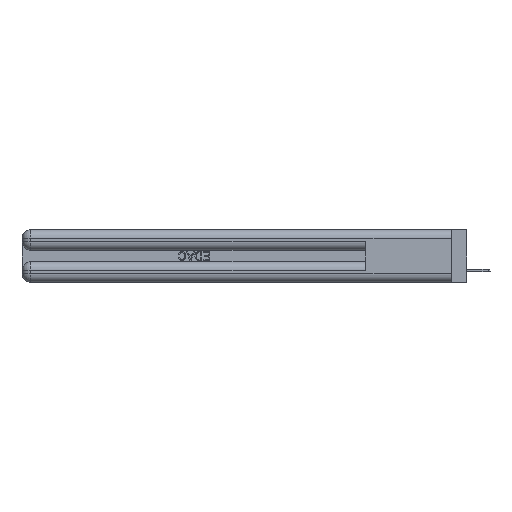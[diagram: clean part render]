
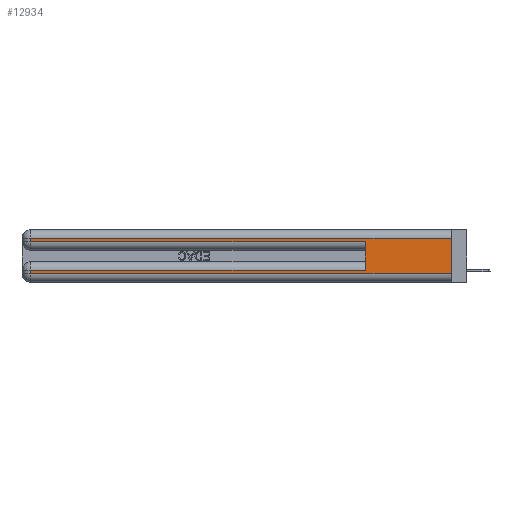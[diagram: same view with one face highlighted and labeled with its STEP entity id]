
A CAD part, left-side view. The second image highlights one B-rep face of the part: STEP entity #12934.
In plain terms, the highlighted planar face has unit normal (-1, 0, 0).
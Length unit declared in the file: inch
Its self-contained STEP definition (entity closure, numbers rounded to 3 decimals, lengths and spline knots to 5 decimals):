
#22 = AXIS2_PLACEMENT_3D ( 'NONE', #28005, #27720, #12625 ) ;
#767 = VECTOR ( 'NONE', #29640, 39.37008 ) ;
#1498 = CARTESIAN_POINT ( 'NONE',  ( 0., 0.6, 0.285 ) ) ;
#1683 = ORIENTED_EDGE ( 'NONE', *, *, #37408, .T. ) ;
#1996 = LINE ( 'NONE', #8530, #46665 ) ;
#2522 = CARTESIAN_POINT ( 'NONE',  ( 0., 0., 0.31 ) ) ;
#2991 = ORIENTED_EDGE ( 'NONE', *, *, #3383, .F. ) ;
#3135 = ORIENTED_EDGE ( 'NONE', *, *, #40833, .F. ) ;
#3327 = VECTOR ( 'NONE', #6158, 39.37008 ) ;
#3383 = EDGE_CURVE ( 'NONE', #21858, #6400, #47282, .T. ) ;
#4470 = LINE ( 'NONE', #31161, #49171 ) ;
#5567 = VERTEX_POINT ( 'NONE', #1498 ) ;
#6158 = DIRECTION ( 'NONE',  ( 0., 0., -1. ) ) ;
#6400 = VERTEX_POINT ( 'NONE', #17814 ) ;
#6963 = CARTESIAN_POINT ( 'NONE',  ( 0., 0.6, 0.145 ) ) ;
#8530 = CARTESIAN_POINT ( 'NONE',  ( 0., 2.94, 0.37 ) ) ;
#11016 = CARTESIAN_POINT ( 'NONE',  ( 0., 2.94, 0.37 ) ) ;
#11525 = CARTESIAN_POINT ( 'NONE',  ( 0., 2.94, 0.085 ) ) ;
#11971 = EDGE_CURVE ( 'NONE', #12400, #48151, #46925, .T. ) ;
#12214 = DIRECTION ( 'NONE',  ( 0., 0., -1. ) ) ;
#12400 = VERTEX_POINT ( 'NONE', #11525 ) ;
#12556 = ORIENTED_EDGE ( 'NONE', *, *, #29020, .T. ) ;
#12625 = DIRECTION ( 'NONE',  ( 0., 0., -1. ) ) ;
#12934 = ADVANCED_FACE ( 'NONE', ( #42698 ), #24465, .F. ) ;
#14293 = LINE ( 'NONE', #35962, #14870 ) ;
#14870 = VECTOR ( 'NONE', #16725, 39.37008 ) ;
#16725 = DIRECTION ( 'NONE',  ( 0., -1., 0. ) ) ;
#16782 = VECTOR ( 'NONE', #26331, 39.37008 ) ;
#17787 = LINE ( 'NONE', #41092, #767 ) ;
#17814 = CARTESIAN_POINT ( 'NONE',  ( 0., 0., 0.06 ) ) ;
#18888 = DIRECTION ( 'NONE',  ( 0., 0., -1. ) ) ;
#19220 = VECTOR ( 'NONE', #18888, 39.37008 ) ;
#21858 = VERTEX_POINT ( 'NONE', #2522 ) ;
#24045 = EDGE_CURVE ( 'NONE', #32483, #24258, #1996, .T. ) ;
#24258 = VERTEX_POINT ( 'NONE', #35124 ) ;
#24414 = DIRECTION ( 'NONE',  ( 0., 1., 0. ) ) ;
#24460 = LINE ( 'NONE', #47608, #30542 ) ;
#24465 = PLANE ( 'NONE',  #22 ) ;
#25417 = CARTESIAN_POINT ( 'NONE',  ( 0., 0., 0.37 ) ) ;
#25487 = EDGE_LOOP ( 'NONE', ( #2991, #12556, #35026, #29604, #3135, #1683, #39627, #26006 ) ) ;
#26006 = ORIENTED_EDGE ( 'NONE', *, *, #37090, .T. ) ;
#26331 = DIRECTION ( 'NONE',  ( 0., 0., 1. ) ) ;
#27024 = CARTESIAN_POINT ( 'NONE',  ( 0., 2.94, 0.06 ) ) ;
#27114 = LINE ( 'NONE', #6963, #16782 ) ;
#27720 = DIRECTION ( 'NONE',  ( 1., 0., 0. ) ) ;
#28005 = CARTESIAN_POINT ( 'NONE',  ( 0., 0., 0.37 ) ) ;
#29020 = EDGE_CURVE ( 'NONE', #21858, #32483, #4470, .T. ) ;
#29604 = ORIENTED_EDGE ( 'NONE', *, *, #37640, .T. ) ;
#29640 = DIRECTION ( 'NONE',  ( 0., -1., 0. ) ) ;
#30542 = VECTOR ( 'NONE', #24414, 39.37008 ) ;
#31161 = CARTESIAN_POINT ( 'NONE',  ( 0., 0., 0.31 ) ) ;
#32483 = VERTEX_POINT ( 'NONE', #37504 ) ;
#35026 = ORIENTED_EDGE ( 'NONE', *, *, #24045, .T. ) ;
#35077 = CARTESIAN_POINT ( 'NONE',  ( 0., 0.6, 0.085 ) ) ;
#35124 = CARTESIAN_POINT ( 'NONE',  ( 0., 2.94, 0.285 ) ) ;
#35163 = DIRECTION ( 'NONE',  ( 0., 1., 0. ) ) ;
#35962 = CARTESIAN_POINT ( 'NONE',  ( 0., 0., 0.06 ) ) ;
#37090 = EDGE_CURVE ( 'NONE', #48151, #6400, #14293, .T. ) ;
#37408 = EDGE_CURVE ( 'NONE', #42700, #12400, #24460, .T. ) ;
#37504 = CARTESIAN_POINT ( 'NONE',  ( 0., 2.94, 0.31 ) ) ;
#37640 = EDGE_CURVE ( 'NONE', #24258, #5567, #17787, .T. ) ;
#39627 = ORIENTED_EDGE ( 'NONE', *, *, #11971, .T. ) ;
#40833 = EDGE_CURVE ( 'NONE', #42700, #5567, #27114, .T. ) ;
#41092 = CARTESIAN_POINT ( 'NONE',  ( 0., 0., 0.285 ) ) ;
#42698 = FACE_OUTER_BOUND ( 'NONE', #25487, .T. ) ;
#42700 = VERTEX_POINT ( 'NONE', #35077 ) ;
#46665 = VECTOR ( 'NONE', #12214, 39.37008 ) ;
#46925 = LINE ( 'NONE', #11016, #19220 ) ;
#47282 = LINE ( 'NONE', #25417, #3327 ) ;
#47608 = CARTESIAN_POINT ( 'NONE',  ( 0., 0., 0.085 ) ) ;
#48151 = VERTEX_POINT ( 'NONE', #27024 ) ;
#49171 = VECTOR ( 'NONE', #35163, 39.37008 ) ;
